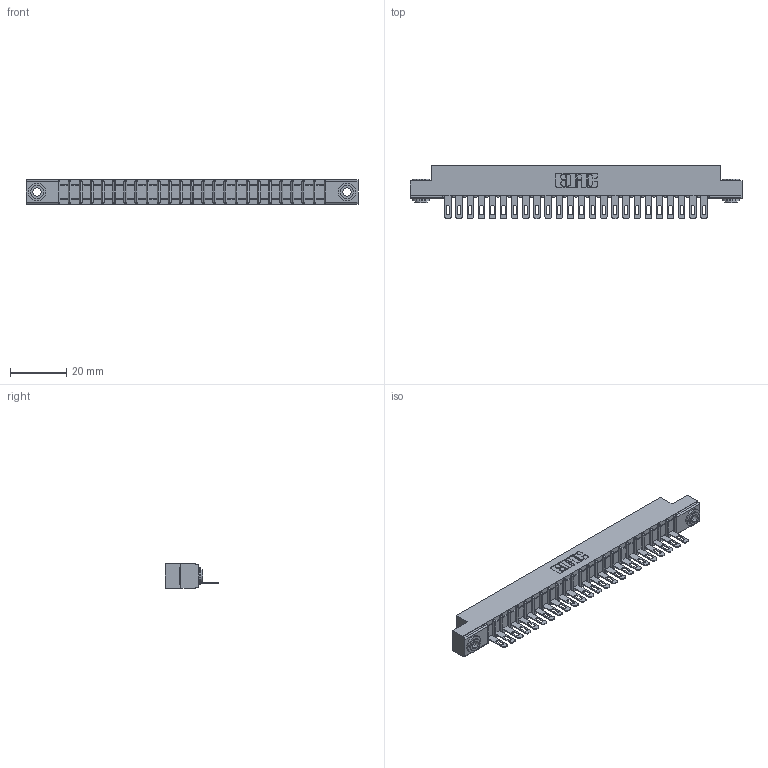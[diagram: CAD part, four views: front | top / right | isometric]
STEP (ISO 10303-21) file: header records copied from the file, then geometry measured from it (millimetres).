
FILE_DESCRIPTION (( 'STEP AP203' ), '1' );
FILE_NAME ('357-024-405-103.STEP', '2020-10-01T11:57:37', ( '' ), ( '' ), 'SwSTEP 2.0', 'SolidWorks 2020', '' );
FILE_SCHEMA (( 'CONFIG_CONTROL_DESIGN' ));
Length unit declared in the file: inch
Products named in the file (4): 307 Part_.156 Dia Mounting Holes; 345-250-002_345-250-002-102; 357-024-405-103; 307-290-001_505
Assembly tree (27 placements, depth 2):
  357-024-405-103
    307 Part_.156 Dia Mounting Holes
    307-290-001_505  x24
    345-250-002_345-250-002-102  x2
Bounding box: 118.11 x 19.18 x 8.71 mm (x, y, z)
Volume: 7485.9 mm3; surface area: 12127 mm2
Topology: 27 solids, 27 shells, 1539 faces, 4323 edges, 2778 vertices
Faces by surface type: plane 958, cylinder 523, sphere 50, cone 8
Entity records: 23833 total; most frequent: CARTESIAN_POINT 3985, ORIENTED_EDGE 3962, DIRECTION 3903, EDGE_CURVE 1981, VECTOR 1503, LINE 1503, VERTEX_POINT 1282, AXIS2_PLACEMENT_3D 1200
